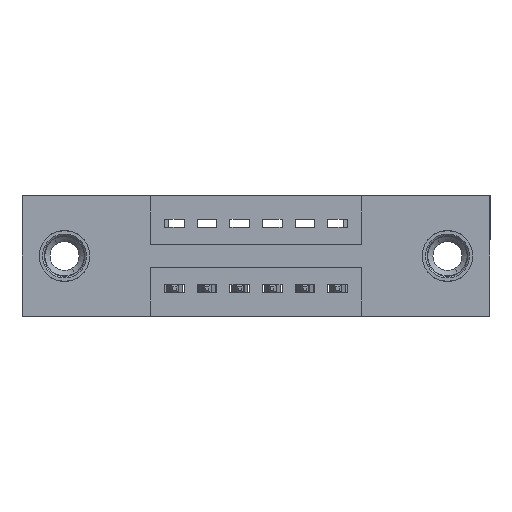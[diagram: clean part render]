
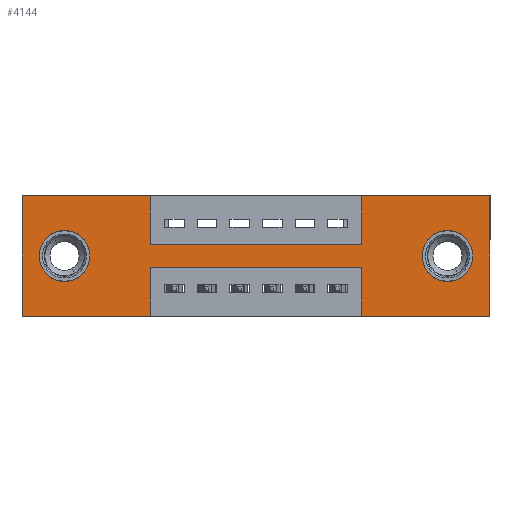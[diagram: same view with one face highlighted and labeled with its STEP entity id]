
A CAD part, front view. The second image highlights one B-rep face of the part: STEP entity #4144.
In plain terms, the highlighted planar face has unit normal (0, -1, 0).
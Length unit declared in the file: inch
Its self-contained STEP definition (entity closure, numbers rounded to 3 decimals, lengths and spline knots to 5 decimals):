
#189 = LINE ( 'NONE', #4622, #1565 ) ;
#221 = DIRECTION ( 'NONE',  ( 0., 0., 1. ) ) ;
#348 = VERTEX_POINT ( 'NONE', #13856 ) ;
#423 = VERTEX_POINT ( 'NONE', #13976 ) ;
#542 = EDGE_CURVE ( 'NONE', #9566, #12265, #14095, .T. ) ;
#582 = EDGE_CURVE ( 'NONE', #12494, #1562, #11541, .T. ) ;
#622 = CARTESIAN_POINT ( 'NONE',  ( 1.0425, 0., -0.37 ) ) ;
#683 = VECTOR ( 'NONE', #1768, 39.37008 ) ;
#749 = CARTESIAN_POINT ( 'NONE',  ( 0., 0., 0. ) ) ;
#942 = DIRECTION ( 'NONE',  ( 0., 0., -1. ) ) ;
#997 = CARTESIAN_POINT ( 'NONE',  ( 0., 0., -0.37 ) ) ;
#1163 = DIRECTION ( 'NONE',  ( 0., 0., -1. ) ) ;
#1316 = LINE ( 'NONE', #4660, #5783 ) ;
#1401 = FACE_BOUND ( 'NONE', #7498, .T. ) ;
#1460 = DIRECTION ( 'NONE',  ( 0., 0., 1. ) ) ;
#1537 = ORIENTED_EDGE ( 'NONE', *, *, #12450, .F. ) ;
#1562 = VERTEX_POINT ( 'NONE', #10508 ) ;
#1565 = VECTOR ( 'NONE', #7843, 39.37008 ) ;
#1750 = DIRECTION ( 'NONE',  ( 0., 0., -1. ) ) ;
#1768 = DIRECTION ( 'NONE',  ( 0., 0., 1. ) ) ;
#1781 = LINE ( 'NONE', #4920, #13053 ) ;
#1971 = ORIENTED_EDGE ( 'NONE', *, *, #13930, .T. ) ;
#2150 = CIRCLE ( 'NONE', #6649, 0.078 ) ;
#2160 = ORIENTED_EDGE ( 'NONE', *, *, #10333, .F. ) ;
#2177 = ORIENTED_EDGE ( 'NONE', *, *, #542, .F. ) ;
#2237 = FACE_OUTER_BOUND ( 'NONE', #7956, .T. ) ;
#2470 = EDGE_CURVE ( 'NONE', #5155, #3789, #4159, .T. ) ;
#2499 = ORIENTED_EDGE ( 'NONE', *, *, #6916, .T. ) ;
#2781 = CARTESIAN_POINT ( 'NONE',  ( 1.305, 0., -0.185 ) ) ;
#3015 = EDGE_CURVE ( 'NONE', #3576, #12602, #11327, .T. ) ;
#3017 = CIRCLE ( 'NONE', #12273, 0.078 ) ;
#3391 = DIRECTION ( 'NONE',  ( 0., 1., 0. ) ) ;
#3513 = VERTEX_POINT ( 'NONE', #6419 ) ;
#3576 = VERTEX_POINT ( 'NONE', #10948 ) ;
#3738 = AXIS2_PLACEMENT_3D ( 'NONE', #10641, #8279, #1750 ) ;
#3761 = CARTESIAN_POINT ( 'NONE',  ( 1.435, 0., -0.37 ) ) ;
#3789 = VERTEX_POINT ( 'NONE', #5673 ) ;
#3810 = EDGE_CURVE ( 'NONE', #12265, #423, #189, .T. ) ;
#3983 = DIRECTION ( 'NONE',  ( -1., 0., 0. ) ) ;
#4130 = DIRECTION ( 'NONE',  ( 1., 0., 0. ) ) ;
#4144 = ADVANCED_FACE ( 'NONE', ( #14047, #1401, #2237 ), #5035, .T. ) ;
#4159 = CIRCLE ( 'NONE', #10689, 0.078 ) ;
#4211 = EDGE_CURVE ( 'NONE', #3513, #13633, #11142, .T. ) ;
#4305 = VECTOR ( 'NONE', #7946, 39.37008 ) ;
#4321 = CARTESIAN_POINT ( 'NONE',  ( 0.3925, 0., -0.15 ) ) ;
#4500 = DIRECTION ( 'NONE',  ( 0., 0., 1. ) ) ;
#4622 = CARTESIAN_POINT ( 'NONE',  ( 0., 0., 0. ) ) ;
#4660 = CARTESIAN_POINT ( 'NONE',  ( 0.3925, 0., 0. ) ) ;
#4663 = EDGE_LOOP ( 'NONE', ( #2499, #4987 ) ) ;
#4714 = DIRECTION ( 'NONE',  ( 0., 0., -1. ) ) ;
#4759 = ORIENTED_EDGE ( 'NONE', *, *, #9152, .F. ) ;
#4851 = VECTOR ( 'NONE', #4714, 39.37008 ) ;
#4920 = CARTESIAN_POINT ( 'NONE',  ( 1.0425, 0., 0. ) ) ;
#4948 = ORIENTED_EDGE ( 'NONE', *, *, #11833, .F. ) ;
#4987 = ORIENTED_EDGE ( 'NONE', *, *, #2470, .T. ) ;
#5035 = PLANE ( 'NONE',  #3738 ) ;
#5155 = VERTEX_POINT ( 'NONE', #7301 ) ;
#5278 = CARTESIAN_POINT ( 'NONE',  ( 1.435, 0., 0. ) ) ;
#5308 = CARTESIAN_POINT ( 'NONE',  ( 0.13, 0., -0.107 ) ) ;
#5487 = LINE ( 'NONE', #622, #683 ) ;
#5649 = CARTESIAN_POINT ( 'NONE',  ( 0.3925, 0., -0.22 ) ) ;
#5673 = CARTESIAN_POINT ( 'NONE',  ( 1.305, 0., -0.107 ) ) ;
#5783 = VECTOR ( 'NONE', #13385, 39.37008 ) ;
#5962 = DIRECTION ( 'NONE',  ( 0., 0., -1. ) ) ;
#6360 = VECTOR ( 'NONE', #9770, 39.37008 ) ;
#6419 = CARTESIAN_POINT ( 'NONE',  ( 1.0425, 0., -0.22 ) ) ;
#6649 = AXIS2_PLACEMENT_3D ( 'NONE', #9928, #3391, #4500 ) ;
#6789 = CARTESIAN_POINT ( 'NONE',  ( 1.305, 0., -0.185 ) ) ;
#6916 = EDGE_CURVE ( 'NONE', #3789, #5155, #3017, .T. ) ;
#6946 = CARTESIAN_POINT ( 'NONE',  ( 0., 0., -0.37 ) ) ;
#6974 = VECTOR ( 'NONE', #4130, 39.37008 ) ;
#6996 = CARTESIAN_POINT ( 'NONE',  ( 0., 0., 0. ) ) ;
#7025 = ORIENTED_EDGE ( 'NONE', *, *, #3810, .F. ) ;
#7082 = DIRECTION ( 'NONE',  ( 0., 1., 0. ) ) ;
#7158 = EDGE_CURVE ( 'NONE', #423, #348, #1316, .T. ) ;
#7214 = CARTESIAN_POINT ( 'NONE',  ( 1.0425, 0., -0.15 ) ) ;
#7249 = ORIENTED_EDGE ( 'NONE', *, *, #582, .T. ) ;
#7301 = CARTESIAN_POINT ( 'NONE',  ( 1.305, 0., -0.263 ) ) ;
#7488 = ORIENTED_EDGE ( 'NONE', *, *, #8747, .F. ) ;
#7498 = EDGE_LOOP ( 'NONE', ( #7249, #1971 ) ) ;
#7553 = CARTESIAN_POINT ( 'NONE',  ( 0., 0., 0. ) ) ;
#7679 = ORIENTED_EDGE ( 'NONE', *, *, #4211, .F. ) ;
#7680 = DIRECTION ( 'NONE',  ( 0., 1., 0. ) ) ;
#7843 = DIRECTION ( 'NONE',  ( 1., 0., 0. ) ) ;
#7946 = DIRECTION ( 'NONE',  ( -1., 0., 0. ) ) ;
#7956 = EDGE_LOOP ( 'NONE', ( #4759, #7679, #9646, #12222, #4948, #13820, #7488, #1537, #12704, #7025, #2177, #2160 ) ) ;
#8065 = LINE ( 'NONE', #10042, #4851 ) ;
#8225 = VECTOR ( 'NONE', #14016, 39.37008 ) ;
#8244 = VERTEX_POINT ( 'NONE', #8952 ) ;
#8279 = DIRECTION ( 'NONE',  ( 0., -1., 0. ) ) ;
#8443 = CARTESIAN_POINT ( 'NONE',  ( 1.0425, 0., -0.37 ) ) ;
#8527 = LINE ( 'NONE', #5278, #13676 ) ;
#8560 = CARTESIAN_POINT ( 'NONE',  ( 0.3925, 0., -0.22 ) ) ;
#8708 = DIRECTION ( 'NONE',  ( 0., 0., 1. ) ) ;
#8747 = EDGE_CURVE ( 'NONE', #9525, #3576, #1781, .T. ) ;
#8823 = AXIS2_PLACEMENT_3D ( 'NONE', #13299, #11099, #221 ) ;
#8952 = CARTESIAN_POINT ( 'NONE',  ( 0.3925, 0., -0.37 ) ) ;
#8960 = VECTOR ( 'NONE', #8708, 39.37008 ) ;
#9152 = EDGE_CURVE ( 'NONE', #13633, #8244, #8065, .T. ) ;
#9365 = VECTOR ( 'NONE', #3983, 39.37008 ) ;
#9525 = VERTEX_POINT ( 'NONE', #7214 ) ;
#9556 = VERTEX_POINT ( 'NONE', #8443 ) ;
#9566 = VERTEX_POINT ( 'NONE', #997 ) ;
#9646 = ORIENTED_EDGE ( 'NONE', *, *, #11771, .F. ) ;
#9770 = DIRECTION ( 'NONE',  ( 1., 0., 0. ) ) ;
#9928 = CARTESIAN_POINT ( 'NONE',  ( 0.13, 0., -0.185 ) ) ;
#10042 = CARTESIAN_POINT ( 'NONE',  ( 0.3925, 0., -0.37 ) ) ;
#10163 = CARTESIAN_POINT ( 'NONE',  ( 1.435, 0., 0. ) ) ;
#10333 = EDGE_CURVE ( 'NONE', #8244, #9566, #13021, .T. ) ;
#10508 = CARTESIAN_POINT ( 'NONE',  ( 0.13, 0., -0.263 ) ) ;
#10641 = CARTESIAN_POINT ( 'NONE',  ( 0., 0., -0.37 ) ) ;
#10689 = AXIS2_PLACEMENT_3D ( 'NONE', #2781, #7082, #5962 ) ;
#10948 = CARTESIAN_POINT ( 'NONE',  ( 1.0425, 0., 0. ) ) ;
#11099 = DIRECTION ( 'NONE',  ( 0., 1., 0. ) ) ;
#11142 = LINE ( 'NONE', #8560, #8225 ) ;
#11327 = LINE ( 'NONE', #749, #6360 ) ;
#11541 = CIRCLE ( 'NONE', #8823, 0.078 ) ;
#11771 = EDGE_CURVE ( 'NONE', #9556, #3513, #5487, .T. ) ;
#11833 = EDGE_CURVE ( 'NONE', #12602, #12248, #8527, .T. ) ;
#12222 = ORIENTED_EDGE ( 'NONE', *, *, #12851, .F. ) ;
#12248 = VERTEX_POINT ( 'NONE', #3761 ) ;
#12265 = VERTEX_POINT ( 'NONE', #6996 ) ;
#12273 = AXIS2_PLACEMENT_3D ( 'NONE', #6789, #7680, #1163 ) ;
#12443 = LINE ( 'NONE', #12805, #9365 ) ;
#12450 = EDGE_CURVE ( 'NONE', #348, #9525, #12785, .T. ) ;
#12494 = VERTEX_POINT ( 'NONE', #5308 ) ;
#12602 = VERTEX_POINT ( 'NONE', #10163 ) ;
#12704 = ORIENTED_EDGE ( 'NONE', *, *, #7158, .F. ) ;
#12785 = LINE ( 'NONE', #4321, #6974 ) ;
#12805 = CARTESIAN_POINT ( 'NONE',  ( 0., 0., -0.37 ) ) ;
#12851 = EDGE_CURVE ( 'NONE', #12248, #9556, #12443, .T. ) ;
#13021 = LINE ( 'NONE', #6946, #4305 ) ;
#13053 = VECTOR ( 'NONE', #1460, 39.37008 ) ;
#13299 = CARTESIAN_POINT ( 'NONE',  ( 0.13, 0., -0.185 ) ) ;
#13385 = DIRECTION ( 'NONE',  ( 0., 0., -1. ) ) ;
#13633 = VERTEX_POINT ( 'NONE', #5649 ) ;
#13676 = VECTOR ( 'NONE', #942, 39.37008 ) ;
#13820 = ORIENTED_EDGE ( 'NONE', *, *, #3015, .F. ) ;
#13856 = CARTESIAN_POINT ( 'NONE',  ( 0.3925, 0., -0.15 ) ) ;
#13930 = EDGE_CURVE ( 'NONE', #1562, #12494, #2150, .T. ) ;
#13976 = CARTESIAN_POINT ( 'NONE',  ( 0.3925, 0., 0. ) ) ;
#14016 = DIRECTION ( 'NONE',  ( -1., 0., 0. ) ) ;
#14047 = FACE_BOUND ( 'NONE', #4663, .T. ) ;
#14095 = LINE ( 'NONE', #7553, #8960 ) ;
